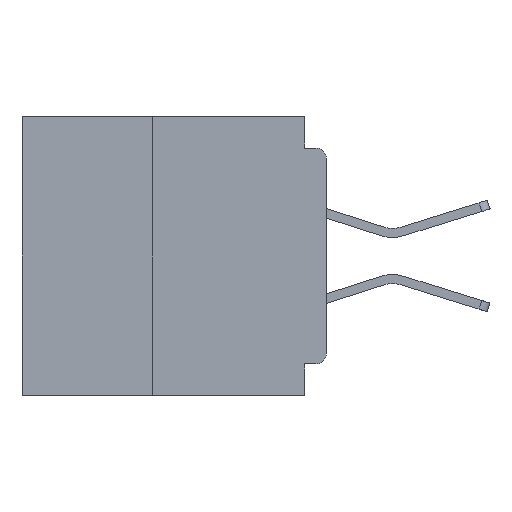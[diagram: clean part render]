
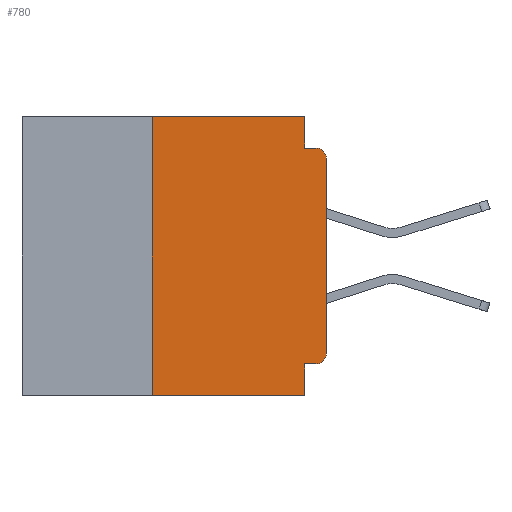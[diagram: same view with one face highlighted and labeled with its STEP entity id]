
A CAD part, left-side view. The second image highlights one B-rep face of the part: STEP entity #780.
In plain terms, the highlighted planar face has unit normal (-1, 0, 0).
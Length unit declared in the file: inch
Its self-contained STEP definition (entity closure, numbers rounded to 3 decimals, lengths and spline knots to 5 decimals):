
#780 = ADVANCED_FACE ( 'NONE', ( #10213 ), #9083, .F. ) ;
#992 = ORIENTED_EDGE ( 'NONE', *, *, #27165, .T. ) ;
#1702 = CIRCLE ( 'NONE', #10326, 0.015 ) ;
#2369 = DIRECTION ( 'NONE',  ( 0., 0., -1. ) ) ;
#3375 = VECTOR ( 'NONE', #46248, 39.37008 ) ;
#3596 = LINE ( 'NONE', #4893, #10091 ) ;
#4893 = CARTESIAN_POINT ( 'NONE',  ( 0., 0.437, -0.4 ) ) ;
#5042 = ORIENTED_EDGE ( 'NONE', *, *, #15594, .T. ) ;
#6612 = DIRECTION ( 'NONE',  ( 0., 0., -1. ) ) ;
#6778 = DIRECTION ( 'NONE',  ( 1., 0., 0. ) ) ;
#7147 = CARTESIAN_POINT ( 'NONE',  ( 0., 0.031, -0.4 ) ) ;
#7945 = CARTESIAN_POINT ( 'NONE',  ( 0., 0.25, -0.4 ) ) ;
#8350 = CARTESIAN_POINT ( 'NONE',  ( 0., 0., -0.045 ) ) ;
#8700 = DIRECTION ( 'NONE',  ( 0., -1., 0. ) ) ;
#8728 = LINE ( 'NONE', #20900, #16450 ) ;
#9083 = PLANE ( 'NONE',  #44684 ) ;
#9138 = CARTESIAN_POINT ( 'NONE',  ( 0., 0.437, 0. ) ) ;
#9322 = EDGE_CURVE ( 'NONE', #30959, #29596, #46449, .T. ) ;
#10014 = EDGE_CURVE ( 'NONE', #30691, #21920, #13457, .T. ) ;
#10091 = VECTOR ( 'NONE', #8700, 39.37008 ) ;
#10164 = EDGE_CURVE ( 'NONE', #17240, #13318, #8728, .T. ) ;
#10213 = FACE_OUTER_BOUND ( 'NONE', #39589, .T. ) ;
#10326 = AXIS2_PLACEMENT_3D ( 'NONE', #22557, #48718, #26313 ) ;
#12124 = DIRECTION ( 'NONE',  ( 0., -1., 0. ) ) ;
#13251 = CARTESIAN_POINT ( 'NONE',  ( 0., 0.25, 0. ) ) ;
#13318 = VERTEX_POINT ( 'NONE', #28753 ) ;
#13457 = LINE ( 'NONE', #31382, #3375 ) ;
#13986 = ORIENTED_EDGE ( 'NONE', *, *, #22308, .F. ) ;
#14104 = ORIENTED_EDGE ( 'NONE', *, *, #14310, .F. ) ;
#14265 = ORIENTED_EDGE ( 'NONE', *, *, #10164, .F. ) ;
#14310 = EDGE_CURVE ( 'NONE', #38546, #30691, #40760, .T. ) ;
#14528 = EDGE_CURVE ( 'NONE', #44155, #21920, #3596, .T. ) ;
#15459 = CARTESIAN_POINT ( 'NONE',  ( 0., 0.015, -0.045 ) ) ;
#15594 = EDGE_CURVE ( 'NONE', #18824, #29596, #1702, .T. ) ;
#15698 = ORIENTED_EDGE ( 'NONE', *, *, #14528, .T. ) ;
#16082 = VECTOR ( 'NONE', #43480, 39.37008 ) ;
#16450 = VECTOR ( 'NONE', #17061, 39.37008 ) ;
#16541 = VECTOR ( 'NONE', #12124, 39.37008 ) ;
#17061 = DIRECTION ( 'NONE',  ( 0., -1., 0. ) ) ;
#17240 = VERTEX_POINT ( 'NONE', #13251 ) ;
#17262 = LINE ( 'NONE', #43320, #16082 ) ;
#17411 = VECTOR ( 'NONE', #45769, 39.37008 ) ;
#18824 = VERTEX_POINT ( 'NONE', #46763 ) ;
#19567 = AXIS2_PLACEMENT_3D ( 'NONE', #47515, #25125, #2369 ) ;
#20900 = CARTESIAN_POINT ( 'NONE',  ( 0., 0.437, 0. ) ) ;
#21920 = VERTEX_POINT ( 'NONE', #7147 ) ;
#22308 = EDGE_CURVE ( 'NONE', #13318, #30959, #17262, .T. ) ;
#22557 = CARTESIAN_POINT ( 'NONE',  ( 0., 0.015, -0.06 ) ) ;
#23470 = CARTESIAN_POINT ( 'NONE',  ( 0., 0., -0.355 ) ) ;
#23491 = ORIENTED_EDGE ( 'NONE', *, *, #10014, .F. ) ;
#25125 = DIRECTION ( 'NONE',  ( -1., 0., 0. ) ) ;
#26313 = DIRECTION ( 'NONE',  ( 0., 0., -1. ) ) ;
#27013 = CIRCLE ( 'NONE', #19567, 0.015 ) ;
#27165 = EDGE_CURVE ( 'NONE', #32195, #18824, #43804, .T. ) ;
#27225 = DIRECTION ( 'NONE',  ( 0., 1., 0. ) ) ;
#27487 = ORIENTED_EDGE ( 'NONE', *, *, #40118, .T. ) ;
#28740 = DIRECTION ( 'NONE',  ( 0., 0., 1. ) ) ;
#28753 = CARTESIAN_POINT ( 'NONE',  ( 0., 0.031, 0. ) ) ;
#29596 = VERTEX_POINT ( 'NONE', #15459 ) ;
#29634 = VECTOR ( 'NONE', #27225, 39.37008 ) ;
#30691 = VERTEX_POINT ( 'NONE', #37057 ) ;
#30959 = VERTEX_POINT ( 'NONE', #38840 ) ;
#31382 = CARTESIAN_POINT ( 'NONE',  ( 0., 0.031, -0.4 ) ) ;
#32195 = VERTEX_POINT ( 'NONE', #34212 ) ;
#32838 = CARTESIAN_POINT ( 'NONE',  ( 0., 0.25, -0.4 ) ) ;
#33665 = ORIENTED_EDGE ( 'NONE', *, *, #9322, .F. ) ;
#33842 = VECTOR ( 'NONE', #28740, 39.37008 ) ;
#34212 = CARTESIAN_POINT ( 'NONE',  ( 0., 0., -0.34 ) ) ;
#34651 = EDGE_CURVE ( 'NONE', #44155, #17240, #37399, .T. ) ;
#35246 = ORIENTED_EDGE ( 'NONE', *, *, #34651, .F. ) ;
#37057 = CARTESIAN_POINT ( 'NONE',  ( 0., 0.031, -0.355 ) ) ;
#37399 = LINE ( 'NONE', #7945, #17411 ) ;
#37537 = CARTESIAN_POINT ( 'NONE',  ( 0., 0.015, -0.355 ) ) ;
#38546 = VERTEX_POINT ( 'NONE', #37537 ) ;
#38840 = CARTESIAN_POINT ( 'NONE',  ( 0., 0.031, -0.045 ) ) ;
#39589 = EDGE_LOOP ( 'NONE', ( #992, #5042, #33665, #13986, #14265, #35246, #15698, #23491, #14104, #27487 ) ) ;
#40118 = EDGE_CURVE ( 'NONE', #38546, #32195, #27013, .T. ) ;
#40760 = LINE ( 'NONE', #23470, #29634 ) ;
#43320 = CARTESIAN_POINT ( 'NONE',  ( 0., 0.031, 0. ) ) ;
#43480 = DIRECTION ( 'NONE',  ( 0., 0., -1. ) ) ;
#43643 = CARTESIAN_POINT ( 'NONE',  ( 0., 0., 0. ) ) ;
#43804 = LINE ( 'NONE', #43643, #33842 ) ;
#44155 = VERTEX_POINT ( 'NONE', #32838 ) ;
#44684 = AXIS2_PLACEMENT_3D ( 'NONE', #9138, #6778, #6612 ) ;
#45769 = DIRECTION ( 'NONE',  ( 0., 0., 1. ) ) ;
#46248 = DIRECTION ( 'NONE',  ( 0., 0., -1. ) ) ;
#46449 = LINE ( 'NONE', #8350, #16541 ) ;
#46763 = CARTESIAN_POINT ( 'NONE',  ( 0., 0., -0.06 ) ) ;
#47515 = CARTESIAN_POINT ( 'NONE',  ( 0., 0.015, -0.34 ) ) ;
#48718 = DIRECTION ( 'NONE',  ( -1., 0., 0. ) ) ;
